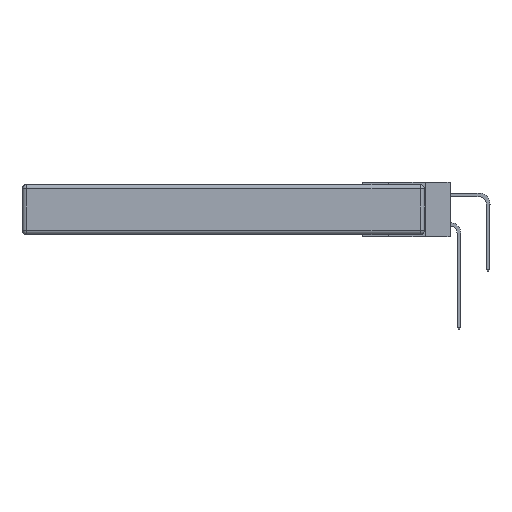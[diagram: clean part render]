
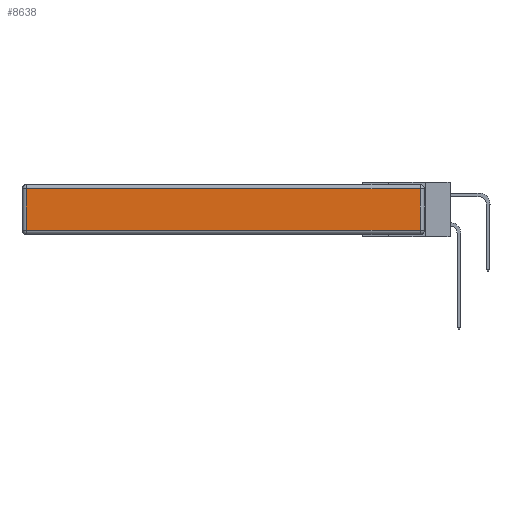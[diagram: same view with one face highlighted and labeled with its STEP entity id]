
A CAD part, left-side view. The second image highlights one B-rep face of the part: STEP entity #8638.
In plain terms, the highlighted planar face has unit normal (-1, 0, 0).
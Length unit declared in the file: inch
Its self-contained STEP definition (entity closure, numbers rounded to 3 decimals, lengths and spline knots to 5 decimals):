
#558 = DIRECTION ( 'NONE',  ( 0., -1., 0. ) ) ;
#568 = LINE ( 'NONE', #14179, #11087 ) ;
#1247 = ORIENTED_EDGE ( 'NONE', *, *, #23938, .T. ) ;
#3138 = VERTEX_POINT ( 'NONE', #15127 ) ;
#3519 = VERTEX_POINT ( 'NONE', #23761 ) ;
#4694 = DIRECTION ( 'NONE',  ( 0., 1., 0. ) ) ;
#5335 = PLANE ( 'NONE',  #9946 ) ;
#5863 = ORIENTED_EDGE ( 'NONE', *, *, #17947, .T. ) ;
#6594 = LINE ( 'NONE', #12721, #17692 ) ;
#8638 = ADVANCED_FACE ( 'NONE', ( #17360 ), #5335, .T. ) ;
#9358 = VERTEX_POINT ( 'NONE', #22061 ) ;
#9510 = EDGE_LOOP ( 'NONE', ( #18705, #10670, #1247, #5863 ) ) ;
#9930 = CARTESIAN_POINT ( 'NONE',  ( 0., 0.03, -0.343 ) ) ;
#9946 = AXIS2_PLACEMENT_3D ( 'NONE', #24269, #11140, #15117 ) ;
#10670 = ORIENTED_EDGE ( 'NONE', *, *, #18469, .T. ) ;
#11087 = VECTOR ( 'NONE', #21689, 39.37008 ) ;
#11140 = DIRECTION ( 'NONE',  ( -1., 0., 0. ) ) ;
#12095 = EDGE_CURVE ( 'NONE', #9358, #3138, #25000, .T. ) ;
#12721 = CARTESIAN_POINT ( 'NONE',  ( 0., 2.75, -0.03 ) ) ;
#14179 = CARTESIAN_POINT ( 'NONE',  ( 0., 2.72, -0.343 ) ) ;
#14736 = VERTEX_POINT ( 'NONE', #17890 ) ;
#15117 = DIRECTION ( 'NONE',  ( 0., 0., 1. ) ) ;
#15127 = CARTESIAN_POINT ( 'NONE',  ( 0., 0.03, -0.313 ) ) ;
#16531 = CARTESIAN_POINT ( 'NONE',  ( 0., 0., -0.313 ) ) ;
#17360 = FACE_OUTER_BOUND ( 'NONE', #9510, .T. ) ;
#17692 = VECTOR ( 'NONE', #4694, 39.37008 ) ;
#17890 = CARTESIAN_POINT ( 'NONE',  ( 0., 2.72, -0.03 ) ) ;
#17947 = EDGE_CURVE ( 'NONE', #14736, #9358, #568, .T. ) ;
#18469 = EDGE_CURVE ( 'NONE', #3138, #3519, #24789, .T. ) ;
#18705 = ORIENTED_EDGE ( 'NONE', *, *, #12095, .T. ) ;
#19070 = VECTOR ( 'NONE', #558, 39.37008 ) ;
#21689 = DIRECTION ( 'NONE',  ( 0., 0., -1. ) ) ;
#22061 = CARTESIAN_POINT ( 'NONE',  ( 0., 2.72, -0.313 ) ) ;
#22605 = VECTOR ( 'NONE', #23876, 39.37008 ) ;
#23761 = CARTESIAN_POINT ( 'NONE',  ( 0., 0.03, -0.03 ) ) ;
#23876 = DIRECTION ( 'NONE',  ( 0., 0., 1. ) ) ;
#23938 = EDGE_CURVE ( 'NONE', #3519, #14736, #6594, .T. ) ;
#24269 = CARTESIAN_POINT ( 'NONE',  ( 0., 0., -0.343 ) ) ;
#24789 = LINE ( 'NONE', #9930, #22605 ) ;
#25000 = LINE ( 'NONE', #16531, #19070 ) ;
